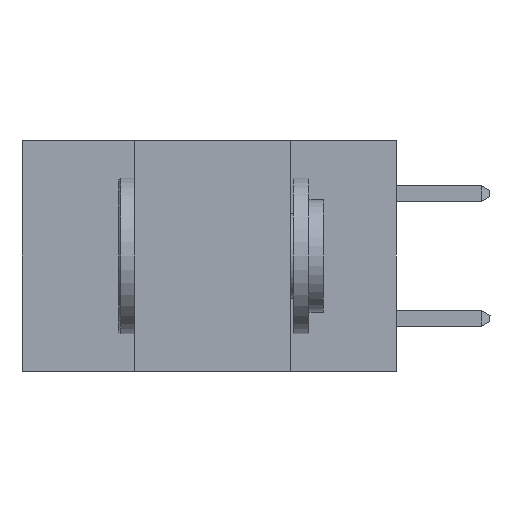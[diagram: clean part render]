
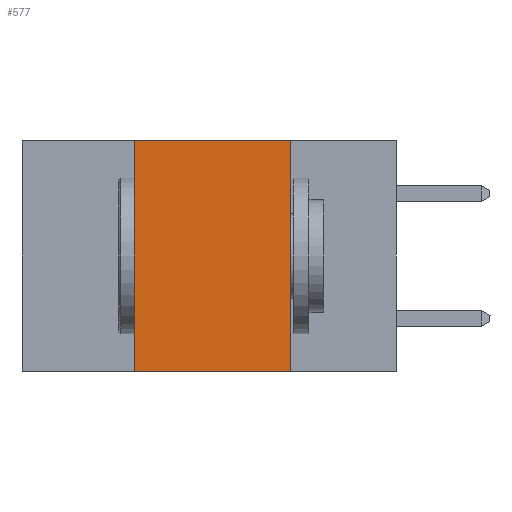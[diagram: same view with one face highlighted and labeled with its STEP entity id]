
A CAD part, left-side view. The second image highlights one B-rep face of the part: STEP entity #577.
In plain terms, the highlighted planar face has unit normal (-1, 0, 0).
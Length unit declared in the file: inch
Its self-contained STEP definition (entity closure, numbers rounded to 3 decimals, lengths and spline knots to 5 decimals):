
#398 = FACE_OUTER_BOUND ( 'NONE', #7867, .T. ) ;
#577 = ADVANCED_FACE ( 'NONE', ( #398 ), #3568, .F. ) ;
#678 = CARTESIAN_POINT ( 'NONE',  ( 0., 0.17, 0. ) ) ;
#1045 = LINE ( 'NONE', #8173, #5659 ) ;
#1184 = DIRECTION ( 'NONE',  ( 0., 0., 1. ) ) ;
#1391 = ORIENTED_EDGE ( 'NONE', *, *, #1696, .F. ) ;
#1696 = EDGE_CURVE ( 'NONE', #5110, #4225, #8142, .T. ) ;
#1763 = DIRECTION ( 'NONE',  ( 0., 0., -1. ) ) ;
#2390 = VERTEX_POINT ( 'NONE', #3161 ) ;
#2472 = EDGE_CURVE ( 'NONE', #5110, #2390, #1045, .T. ) ;
#2741 = VECTOR ( 'NONE', #1763, 39.37008 ) ;
#3161 = CARTESIAN_POINT ( 'NONE',  ( 0., 0.17, -0.37 ) ) ;
#3531 = CARTESIAN_POINT ( 'NONE',  ( 0., 0.42, -0.37 ) ) ;
#3568 = PLANE ( 'NONE',  #5947 ) ;
#3732 = CARTESIAN_POINT ( 'NONE',  ( 0., 0.6, 0. ) ) ;
#3900 = VECTOR ( 'NONE', #1184, 39.37008 ) ;
#3910 = DIRECTION ( 'NONE',  ( 0., 0., -1. ) ) ;
#4225 = VERTEX_POINT ( 'NONE', #8024 ) ;
#4375 = CARTESIAN_POINT ( 'NONE',  ( 0., 0.6, 0. ) ) ;
#4889 = DIRECTION ( 'NONE',  ( 1., 0., 0. ) ) ;
#4892 = LINE ( 'NONE', #9687, #2741 ) ;
#5110 = VERTEX_POINT ( 'NONE', #8949 ) ;
#5659 = VECTOR ( 'NONE', #8160, 39.37008 ) ;
#5940 = VERTEX_POINT ( 'NONE', #678 ) ;
#5947 = AXIS2_PLACEMENT_3D ( 'NONE', #3732, #4889, #3910 ) ;
#6249 = ORIENTED_EDGE ( 'NONE', *, *, #6898, .F. ) ;
#6562 = VECTOR ( 'NONE', #9117, 39.37008 ) ;
#6879 = ORIENTED_EDGE ( 'NONE', *, *, #2472, .T. ) ;
#6898 = EDGE_CURVE ( 'NONE', #4225, #5940, #7068, .T. ) ;
#7068 = LINE ( 'NONE', #4375, #6562 ) ;
#7867 = EDGE_LOOP ( 'NONE', ( #9633, #6249, #1391, #6879 ) ) ;
#8024 = CARTESIAN_POINT ( 'NONE',  ( 0., 0.42, 0. ) ) ;
#8142 = LINE ( 'NONE', #3531, #3900 ) ;
#8160 = DIRECTION ( 'NONE',  ( 0., -1., 0. ) ) ;
#8173 = CARTESIAN_POINT ( 'NONE',  ( 0., 0.6, -0.37 ) ) ;
#8949 = CARTESIAN_POINT ( 'NONE',  ( 0., 0.42, -0.37 ) ) ;
#9117 = DIRECTION ( 'NONE',  ( 0., -1., 0. ) ) ;
#9396 = EDGE_CURVE ( 'NONE', #5940, #2390, #4892, .T. ) ;
#9633 = ORIENTED_EDGE ( 'NONE', *, *, #9396, .F. ) ;
#9687 = CARTESIAN_POINT ( 'NONE',  ( 0., 0.17, -0.37 ) ) ;
